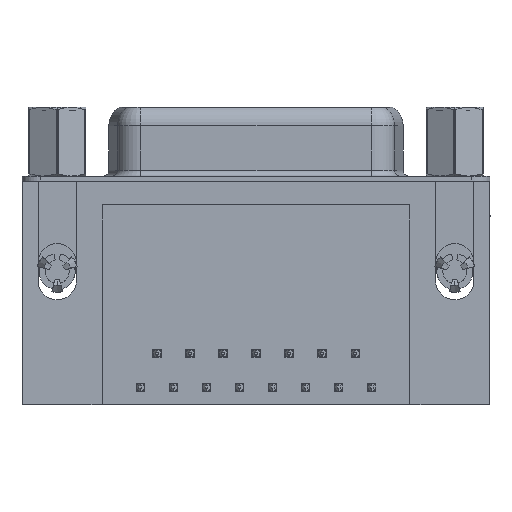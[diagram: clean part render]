
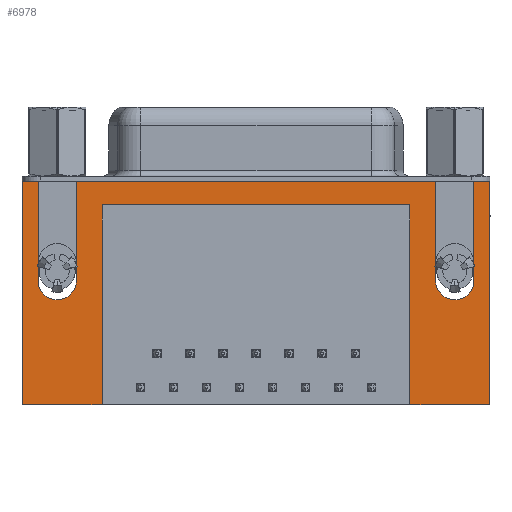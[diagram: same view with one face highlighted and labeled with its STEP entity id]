
A CAD part, front view. The second image highlights one B-rep face of the part: STEP entity #6978.
In plain terms, the highlighted planar face has unit normal (0, -1, 0).
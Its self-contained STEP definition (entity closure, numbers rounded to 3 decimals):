
#208 = VERTEX_POINT ( 'NONE', #18795 ) ;
#354 = VERTEX_POINT ( 'NONE', #24876 ) ;
#788 = LINE ( 'NONE', #19573, #12786 ) ;
#1156 = DIRECTION ( 'NONE',  ( -1., 0., 0. ) ) ;
#1297 = DIRECTION ( 'NONE',  ( 0., -1., 0. ) ) ;
#1416 = VERTEX_POINT ( 'NONE', #12612 ) ;
#1525 = DIRECTION ( 'NONE',  ( 0., 0., -1. ) ) ;
#1561 = ORIENTED_EDGE ( 'NONE', *, *, #1786, .T. ) ;
#1786 = EDGE_CURVE ( 'NONE', #8787, #28636, #27115, .T. ) ;
#1803 = ORIENTED_EDGE ( 'NONE', *, *, #6572, .F. ) ;
#2200 = VERTEX_POINT ( 'NONE', #22406 ) ;
#3187 = CARTESIAN_POINT ( 'NONE',  ( 31.72, -6.275, -8.35 ) ) ;
#3389 = VECTOR ( 'NONE', #14851, 1000. ) ;
#3396 = LINE ( 'NONE', #16795, #10180 ) ;
#3443 = EDGE_CURVE ( 'NONE', #8787, #25249, #21406, .T. ) ;
#3561 = DIRECTION ( 'NONE',  ( 0., 0., -1. ) ) ;
#4194 = LINE ( 'NONE', #27637, #3389 ) ;
#4384 = VECTOR ( 'NONE', #29145, 1000. ) ;
#4876 = CIRCLE ( 'NONE', #28567, 1.6 ) ;
#5974 = VERTEX_POINT ( 'NONE', #24509 ) ;
#6107 = PLANE ( 'NONE',  #22365 ) ;
#6183 = VECTOR ( 'NONE', #24067, 1000. ) ;
#6202 = VECTOR ( 'NONE', #16627, 1000. ) ;
#6329 = ORIENTED_EDGE ( 'NONE', *, *, #7038, .F. ) ;
#6460 = CARTESIAN_POINT ( 'NONE',  ( -1.6, -6.275, 0. ) ) ;
#6572 = EDGE_CURVE ( 'NONE', #21184, #2200, #18134, .T. ) ;
#6944 = EDGE_CURVE ( 'NONE', #7426, #208, #8474, .T. ) ;
#6978 = ADVANCED_FACE ( 'NONE', ( #9276 ), #6107, .T. ) ;
#6999 = CARTESIAN_POINT ( 'NONE',  ( 3.765, -6.275, -18.76 ) ) ;
#7038 = EDGE_CURVE ( 'NONE', #12578, #9368, #19687, .T. ) ;
#7141 = VERTEX_POINT ( 'NONE', #9554 ) ;
#7426 = VERTEX_POINT ( 'NONE', #3187 ) ;
#7459 = CARTESIAN_POINT ( 'NONE',  ( -1.6, -6.275, -8.35 ) ) ;
#8474 = CIRCLE ( 'NONE', #13790, 1.6 ) ;
#8787 = VERTEX_POINT ( 'NONE', #15792 ) ;
#8972 = EDGE_CURVE ( 'NONE', #26055, #7141, #24787, .T. ) ;
#9112 = LINE ( 'NONE', #19061, #23546 ) ;
#9276 = FACE_OUTER_BOUND ( 'NONE', #31934, .T. ) ;
#9368 = VERTEX_POINT ( 'NONE', #7459 ) ;
#9554 = CARTESIAN_POINT ( 'NONE',  ( 31.72, -6.275, 0. ) ) ;
#9574 = VECTOR ( 'NONE', #20124, 1000. ) ;
#10180 = VECTOR ( 'NONE', #32175, 1000. ) ;
#10622 = EDGE_CURVE ( 'NONE', #7141, #7426, #3396, .T. ) ;
#10916 = CARTESIAN_POINT ( 'NONE',  ( 33.32, -6.275, -8.35 ) ) ;
#11233 = DIRECTION ( 'NONE',  ( 0., 0., -1. ) ) ;
#12578 = VERTEX_POINT ( 'NONE', #6460 ) ;
#12612 = CARTESIAN_POINT ( 'NONE',  ( -2.935, -6.275, -18.76 ) ) ;
#12786 = VECTOR ( 'NONE', #29816, 1000. ) ;
#12840 = VERTEX_POINT ( 'NONE', #6999 ) ;
#13244 = EDGE_CURVE ( 'NONE', #9368, #354, #4876, .T. ) ;
#13480 = VECTOR ( 'NONE', #32490, 1000. ) ;
#13505 = DIRECTION ( 'NONE',  ( -1., 0., 0. ) ) ;
#13790 = AXIS2_PLACEMENT_3D ( 'NONE', #10916, #28890, #13505 ) ;
#13855 = ORIENTED_EDGE ( 'NONE', *, *, #26507, .F. ) ;
#14044 = CARTESIAN_POINT ( 'NONE',  ( 36.255, -6.275, 0. ) ) ;
#14334 = DIRECTION ( 'NONE',  ( 1., 0., 0. ) ) ;
#14383 = ORIENTED_EDGE ( 'NONE', *, *, #13244, .F. ) ;
#14741 = VECTOR ( 'NONE', #16287, 1000. ) ;
#14851 = DIRECTION ( 'NONE',  ( 0., 0., 1. ) ) ;
#14984 = CARTESIAN_POINT ( 'NONE',  ( 1.6, -6.275, 0. ) ) ;
#15792 = CARTESIAN_POINT ( 'NONE',  ( 36.255, -6.275, -18.76 ) ) ;
#16287 = DIRECTION ( 'NONE',  ( 1., 0., 0. ) ) ;
#16397 = CARTESIAN_POINT ( 'NONE',  ( -2.935, -6.275, 0. ) ) ;
#16401 = LINE ( 'NONE', #14984, #9574 ) ;
#16552 = CARTESIAN_POINT ( 'NONE',  ( 1.6, -6.275, 0. ) ) ;
#16622 = CARTESIAN_POINT ( 'NONE',  ( 0., -6.275, -8.35 ) ) ;
#16627 = DIRECTION ( 'NONE',  ( 0., 0., 1. ) ) ;
#16674 = CARTESIAN_POINT ( 'NONE',  ( 3.765, -6.275, -2. ) ) ;
#16795 = CARTESIAN_POINT ( 'NONE',  ( 31.72, -6.275, 0. ) ) ;
#17594 = EDGE_CURVE ( 'NONE', #12840, #1416, #9112, .T. ) ;
#17889 = ORIENTED_EDGE ( 'NONE', *, *, #31951, .F. ) ;
#18134 = LINE ( 'NONE', #16674, #24126 ) ;
#18795 = CARTESIAN_POINT ( 'NONE',  ( 34.92, -6.275, -8.35 ) ) ;
#19061 = CARTESIAN_POINT ( 'NONE',  ( 36.255, -6.275, -18.76 ) ) ;
#19191 = VECTOR ( 'NONE', #3561, 1000. ) ;
#19195 = DIRECTION ( 'NONE',  ( 1., 0., 0. ) ) ;
#19422 = CARTESIAN_POINT ( 'NONE',  ( -1.6, -6.275, 0. ) ) ;
#19512 = CARTESIAN_POINT ( 'NONE',  ( 29.555, -6.275, -18.76 ) ) ;
#19573 = CARTESIAN_POINT ( 'NONE',  ( -2.935, -6.275, -2.5 ) ) ;
#19687 = LINE ( 'NONE', #19422, #26526 ) ;
#19817 = LINE ( 'NONE', #29430, #6202 ) ;
#19981 = LINE ( 'NONE', #23926, #19191 ) ;
#20124 = DIRECTION ( 'NONE',  ( 0., 0., 1. ) ) ;
#21184 = VERTEX_POINT ( 'NONE', #24709 ) ;
#21296 = VECTOR ( 'NONE', #14334, 1000. ) ;
#21309 = CARTESIAN_POINT ( 'NONE',  ( 34.92, -6.275, 0. ) ) ;
#21406 = LINE ( 'NONE', #21470, #6183 ) ;
#21470 = CARTESIAN_POINT ( 'NONE',  ( 36.255, -6.275, -18.76 ) ) ;
#21607 = EDGE_CURVE ( 'NONE', #25249, #21184, #19817, .T. ) ;
#21757 = ORIENTED_EDGE ( 'NONE', *, *, #24217, .F. ) ;
#22066 = EDGE_CURVE ( 'NONE', #208, #31883, #4194, .T. ) ;
#22365 = AXIS2_PLACEMENT_3D ( 'NONE', #24029, #26624, #11233 ) ;
#22387 = ORIENTED_EDGE ( 'NONE', *, *, #6944, .F. ) ;
#22406 = CARTESIAN_POINT ( 'NONE',  ( 3.765, -6.275, -2. ) ) ;
#22832 = ORIENTED_EDGE ( 'NONE', *, *, #22066, .F. ) ;
#23546 = VECTOR ( 'NONE', #1156, 1000. ) ;
#23926 = CARTESIAN_POINT ( 'NONE',  ( 3.765, -6.275, -2. ) ) ;
#23958 = CARTESIAN_POINT ( 'NONE',  ( -2.935, -6.275, 0. ) ) ;
#24029 = CARTESIAN_POINT ( 'NONE',  ( -2.935, -6.275, -2.5 ) ) ;
#24067 = DIRECTION ( 'NONE',  ( -1., 0., 0. ) ) ;
#24126 = VECTOR ( 'NONE', #26981, 1000. ) ;
#24217 = EDGE_CURVE ( 'NONE', #5974, #12578, #26537, .T. ) ;
#24509 = CARTESIAN_POINT ( 'NONE',  ( -2.935, -6.275, 0. ) ) ;
#24541 = ORIENTED_EDGE ( 'NONE', *, *, #26341, .F. ) ;
#24709 = CARTESIAN_POINT ( 'NONE',  ( 29.555, -6.275, -2. ) ) ;
#24787 = LINE ( 'NONE', #23958, #4384 ) ;
#24876 = CARTESIAN_POINT ( 'NONE',  ( 1.6, -6.275, -8.35 ) ) ;
#25249 = VERTEX_POINT ( 'NONE', #19512 ) ;
#25880 = ORIENTED_EDGE ( 'NONE', *, *, #10622, .F. ) ;
#26055 = VERTEX_POINT ( 'NONE', #16552 ) ;
#26341 = EDGE_CURVE ( 'NONE', #354, #26055, #16401, .T. ) ;
#26507 = EDGE_CURVE ( 'NONE', #2200, #12840, #19981, .T. ) ;
#26526 = VECTOR ( 'NONE', #1525, 1000. ) ;
#26537 = LINE ( 'NONE', #32296, #21296 ) ;
#26624 = DIRECTION ( 'NONE',  ( 0., -1., 0. ) ) ;
#26957 = ORIENTED_EDGE ( 'NONE', *, *, #21607, .F. ) ;
#26981 = DIRECTION ( 'NONE',  ( -1., 0., 0. ) ) ;
#27115 = LINE ( 'NONE', #33105, #13480 ) ;
#27537 = ORIENTED_EDGE ( 'NONE', *, *, #31071, .F. ) ;
#27637 = CARTESIAN_POINT ( 'NONE',  ( 34.92, -6.275, 0. ) ) ;
#28567 = AXIS2_PLACEMENT_3D ( 'NONE', #16622, #1297, #19195 ) ;
#28636 = VERTEX_POINT ( 'NONE', #14044 ) ;
#28890 = DIRECTION ( 'NONE',  ( 0., -1., 0. ) ) ;
#29145 = DIRECTION ( 'NONE',  ( 1., 0., 0. ) ) ;
#29430 = CARTESIAN_POINT ( 'NONE',  ( 29.555, -6.275, -2. ) ) ;
#29795 = ORIENTED_EDGE ( 'NONE', *, *, #17594, .F. ) ;
#29816 = DIRECTION ( 'NONE',  ( 0., 0., 1. ) ) ;
#30023 = LINE ( 'NONE', #16397, #14741 ) ;
#31071 = EDGE_CURVE ( 'NONE', #1416, #5974, #788, .T. ) ;
#31353 = ORIENTED_EDGE ( 'NONE', *, *, #3443, .F. ) ;
#31883 = VERTEX_POINT ( 'NONE', #21309 ) ;
#31934 = EDGE_LOOP ( 'NONE', ( #22832, #22387, #25880, #32282, #24541, #14383, #6329, #21757, #27537, #29795, #13855, #1803, #26957, #31353, #1561, #17889 ) ) ;
#31951 = EDGE_CURVE ( 'NONE', #31883, #28636, #30023, .T. ) ;
#32175 = DIRECTION ( 'NONE',  ( 0., 0., -1. ) ) ;
#32282 = ORIENTED_EDGE ( 'NONE', *, *, #8972, .F. ) ;
#32296 = CARTESIAN_POINT ( 'NONE',  ( -2.935, -6.275, 0. ) ) ;
#32490 = DIRECTION ( 'NONE',  ( 0., 0., 1. ) ) ;
#33105 = CARTESIAN_POINT ( 'NONE',  ( 36.255, -6.275, -2.5 ) ) ;
